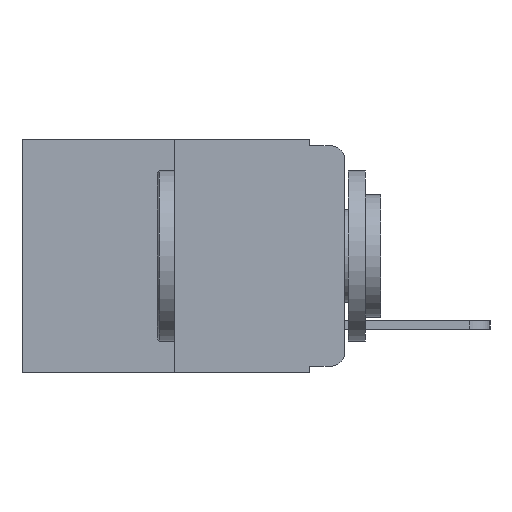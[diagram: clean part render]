
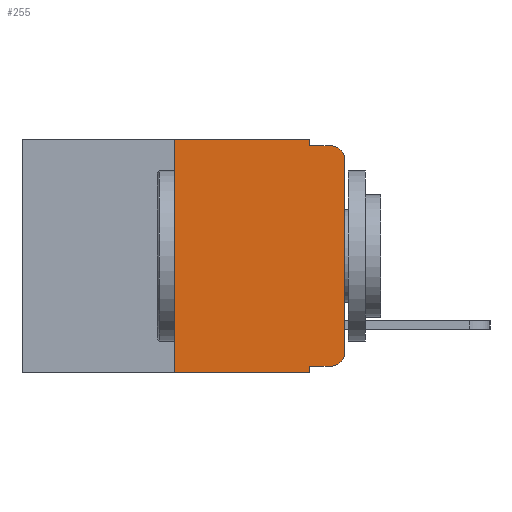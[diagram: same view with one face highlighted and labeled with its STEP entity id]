
A CAD part, left-side view. The second image highlights one B-rep face of the part: STEP entity #255.
In plain terms, the highlighted planar face has unit normal (-1, 0, 0).
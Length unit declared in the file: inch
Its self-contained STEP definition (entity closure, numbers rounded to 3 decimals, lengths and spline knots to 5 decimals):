
#129 = VERTEX_POINT ( 'NONE', #4276 ) ;
#172 = AXIS2_PLACEMENT_3D ( 'NONE', #5740, #6592, #6135 ) ;
#248 = EDGE_LOOP ( 'NONE', ( #4655, #5164, #5219, #5398, #5424, #5919, #5990, #6217, #6301, #6740 ) ) ;
#255 = ADVANCED_FACE ( 'NONE', ( #10057 ), #6121, .F. ) ;
#1302 = AXIS2_PLACEMENT_3D ( 'NONE', #3660, #6771, #6768 ) ;
#1330 = AXIS2_PLACEMENT_3D ( 'NONE', #10798, #3592, #2952 ) ;
#1738 = LINE ( 'NONE', #11617, #7061 ) ;
#1803 = VERTEX_POINT ( 'NONE', #3934 ) ;
#2047 = VECTOR ( 'NONE', #6703, 39.37008 ) ;
#2134 = CARTESIAN_POINT ( 'NONE',  ( 0., 0.051, -0.333 ) ) ;
#2388 = LINE ( 'NONE', #11936, #2047 ) ;
#2741 = LINE ( 'NONE', #2134, #11651 ) ;
#2918 = VERTEX_POINT ( 'NONE', #4270 ) ;
#2952 = DIRECTION ( 'NONE',  ( 0., 0., -1. ) ) ;
#3592 = DIRECTION ( 'NONE',  ( -1., 0., 0. ) ) ;
#3660 = CARTESIAN_POINT ( 'NONE',  ( 0., 0.02, -0.313 ) ) ;
#3910 = EDGE_CURVE ( 'NONE', #9203, #9958, #6137, .T. ) ;
#3934 = CARTESIAN_POINT ( 'NONE',  ( 0., 0., -0.313 ) ) ;
#4195 = EDGE_CURVE ( 'NONE', #1803, #5301, #10423, .T. ) ;
#4209 = EDGE_CURVE ( 'NONE', #5301, #2918, #7737, .T. ) ;
#4210 = EDGE_CURVE ( 'NONE', #7126, #2918, #2388, .T. ) ;
#4235 = EDGE_CURVE ( 'NONE', #11463, #7126, #12175, .T. ) ;
#4236 = EDGE_CURVE ( 'NONE', #9203, #11308, #7400, .T. ) ;
#4237 = EDGE_CURVE ( 'NONE', #4852, #9958, #1738, .T. ) ;
#4250 = EDGE_CURVE ( 'NONE', #4852, #129, #2741, .T. ) ;
#4254 = EDGE_CURVE ( 'NONE', #129, #1803, #9603, .T. ) ;
#4270 = CARTESIAN_POINT ( 'NONE',  ( 0., 0.02, -0.01 ) ) ;
#4276 = CARTESIAN_POINT ( 'NONE',  ( 0., 0.02, -0.333 ) ) ;
#4306 = DIRECTION ( 'NONE',  ( 0., -1., 0. ) ) ;
#4650 = VECTOR ( 'NONE', #5782, 39.37008 ) ;
#4655 = ORIENTED_EDGE ( 'NONE', *, *, #4195, .T. ) ;
#4852 = VERTEX_POINT ( 'NONE', #12756 ) ;
#5164 = ORIENTED_EDGE ( 'NONE', *, *, #4209, .T. ) ;
#5219 = ORIENTED_EDGE ( 'NONE', *, *, #4210, .F. ) ;
#5264 = CARTESIAN_POINT ( 'NONE',  ( 0., 0.051, -0.01 ) ) ;
#5301 = VERTEX_POINT ( 'NONE', #12125 ) ;
#5398 = ORIENTED_EDGE ( 'NONE', *, *, #4235, .F. ) ;
#5413 = EDGE_CURVE ( 'NONE', #11308, #11463, #10644, .T. ) ;
#5424 = ORIENTED_EDGE ( 'NONE', *, *, #5413, .F. ) ;
#5740 = CARTESIAN_POINT ( 'NONE',  ( 0., 0.473, 0. ) ) ;
#5782 = DIRECTION ( 'NONE',  ( 0., 0., -1. ) ) ;
#5919 = ORIENTED_EDGE ( 'NONE', *, *, #4236, .F. ) ;
#5990 = ORIENTED_EDGE ( 'NONE', *, *, #3910, .T. ) ;
#6019 = CARTESIAN_POINT ( 'NONE',  ( 0., 0.051, 0. ) ) ;
#6121 = PLANE ( 'NONE',  #172 ) ;
#6135 = DIRECTION ( 'NONE',  ( 0., 0., -1. ) ) ;
#6137 = LINE ( 'NONE', #10058, #10816 ) ;
#6217 = ORIENTED_EDGE ( 'NONE', *, *, #4237, .F. ) ;
#6301 = ORIENTED_EDGE ( 'NONE', *, *, #4250, .T. ) ;
#6587 = CARTESIAN_POINT ( 'NONE',  ( 0., 0., 0. ) ) ;
#6592 = DIRECTION ( 'NONE',  ( 1., 0., 0. ) ) ;
#6703 = DIRECTION ( 'NONE',  ( 0., -1., 0. ) ) ;
#6737 = DIRECTION ( 'NONE',  ( 0., 0., 1. ) ) ;
#6740 = ORIENTED_EDGE ( 'NONE', *, *, #4254, .T. ) ;
#6768 = DIRECTION ( 'NONE',  ( 0., 0., -1. ) ) ;
#6771 = DIRECTION ( 'NONE',  ( -1., 0., 0. ) ) ;
#7061 = VECTOR ( 'NONE', #7093, 39.37008 ) ;
#7093 = DIRECTION ( 'NONE',  ( 0., 0., -1. ) ) ;
#7126 = VERTEX_POINT ( 'NONE', #5264 ) ;
#7287 = CARTESIAN_POINT ( 'NONE',  ( 0., 0.051, 0. ) ) ;
#7400 = LINE ( 'NONE', #10583, #11913 ) ;
#7737 = CIRCLE ( 'NONE', #1330, 0.02 ) ;
#8026 = VECTOR ( 'NONE', #6737, 39.37008 ) ;
#8391 = CARTESIAN_POINT ( 'NONE',  ( 0., 0.473, 0. ) ) ;
#8890 = CARTESIAN_POINT ( 'NONE',  ( 0., 0.25, 0. ) ) ;
#9203 = VERTEX_POINT ( 'NONE', #9967 ) ;
#9375 = DIRECTION ( 'NONE',  ( 0., -1., 0. ) ) ;
#9603 = CIRCLE ( 'NONE', #1302, 0.02 ) ;
#9958 = VERTEX_POINT ( 'NONE', #10939 ) ;
#9967 = CARTESIAN_POINT ( 'NONE',  ( 0., 0.25, -0.343 ) ) ;
#10057 = FACE_OUTER_BOUND ( 'NONE', #248, .T. ) ;
#10058 = CARTESIAN_POINT ( 'NONE',  ( 0., 0.473, -0.343 ) ) ;
#10423 = LINE ( 'NONE', #6587, #8026 ) ;
#10583 = CARTESIAN_POINT ( 'NONE',  ( 0., 0.25, 0. ) ) ;
#10644 = LINE ( 'NONE', #8391, #12700 ) ;
#10798 = CARTESIAN_POINT ( 'NONE',  ( 0., 0.02, -0.03 ) ) ;
#10816 = VECTOR ( 'NONE', #11872, 39.37008 ) ;
#10939 = CARTESIAN_POINT ( 'NONE',  ( 0., 0.051, -0.343 ) ) ;
#11308 = VERTEX_POINT ( 'NONE', #8890 ) ;
#11463 = VERTEX_POINT ( 'NONE', #7287 ) ;
#11617 = CARTESIAN_POINT ( 'NONE',  ( 0., 0.051, 0. ) ) ;
#11651 = VECTOR ( 'NONE', #4306, 39.37008 ) ;
#11849 = DIRECTION ( 'NONE',  ( 0., 0., 1. ) ) ;
#11872 = DIRECTION ( 'NONE',  ( 0., -1., 0. ) ) ;
#11913 = VECTOR ( 'NONE', #11849, 39.37008 ) ;
#11936 = CARTESIAN_POINT ( 'NONE',  ( 0., 0.051, -0.01 ) ) ;
#12125 = CARTESIAN_POINT ( 'NONE',  ( 0., 0., -0.03 ) ) ;
#12175 = LINE ( 'NONE', #6019, #4650 ) ;
#12700 = VECTOR ( 'NONE', #9375, 39.37008 ) ;
#12756 = CARTESIAN_POINT ( 'NONE',  ( 0., 0.051, -0.333 ) ) ;
